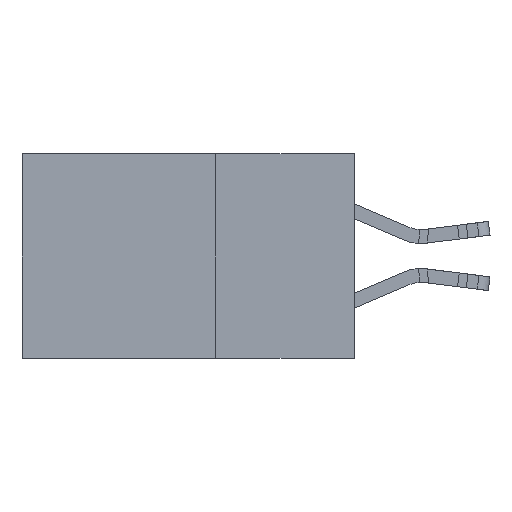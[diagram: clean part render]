
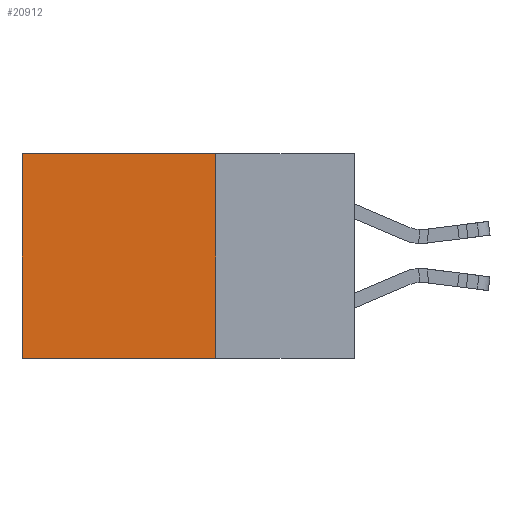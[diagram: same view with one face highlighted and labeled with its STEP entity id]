
A CAD part, left-side view. The second image highlights one B-rep face of the part: STEP entity #20912.
In plain terms, the highlighted planar face has unit normal (-1, 0, 0).
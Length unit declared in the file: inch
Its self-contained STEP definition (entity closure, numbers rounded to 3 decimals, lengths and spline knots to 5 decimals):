
#80 = VERTEX_POINT ( 'NONE', #6116 ) ;
#384 = LINE ( 'NONE', #6016, #4370 ) ;
#1955 = PLANE ( 'NONE',  #20661 ) ;
#1996 = VERTEX_POINT ( 'NONE', #16649 ) ;
#4211 = CARTESIAN_POINT ( 'NONE',  ( 0.2615, 0.25, 0. ) ) ;
#4322 = LINE ( 'NONE', #22541, #17549 ) ;
#4370 = VECTOR ( 'NONE', #15210, 39.37008 ) ;
#4405 = LINE ( 'NONE', #13364, #9918 ) ;
#5443 = FACE_OUTER_BOUND ( 'NONE', #13372, .T. ) ;
#6016 = CARTESIAN_POINT ( 'NONE',  ( 0.2615, 0.25, -0.37 ) ) ;
#6116 = CARTESIAN_POINT ( 'NONE',  ( 0.2615, 0.25, -0.37 ) ) ;
#7510 = CARTESIAN_POINT ( 'NONE',  ( 0.2615, 0.25, -0.37 ) ) ;
#7964 = DIRECTION ( 'NONE',  ( 0., 1., 0. ) ) ;
#8006 = VERTEX_POINT ( 'NONE', #10731 ) ;
#9540 = ORIENTED_EDGE ( 'NONE', *, *, #21520, .T. ) ;
#9557 = CARTESIAN_POINT ( 'NONE',  ( 0.2615, 0.25, 0. ) ) ;
#9918 = VECTOR ( 'NONE', #19125, 39.37008 ) ;
#10367 = ORIENTED_EDGE ( 'NONE', *, *, #22937, .T. ) ;
#10731 = CARTESIAN_POINT ( 'NONE',  ( 0.2615, 0.6, -0.37 ) ) ;
#13364 = CARTESIAN_POINT ( 'NONE',  ( 0.2615, 0.25, -0.37 ) ) ;
#13372 = EDGE_LOOP ( 'NONE', ( #9540, #13458, #20844, #10367 ) ) ;
#13458 = ORIENTED_EDGE ( 'NONE', *, *, #15633, .F. ) ;
#14982 = DIRECTION ( 'NONE',  ( 1., 0., 0. ) ) ;
#15204 = LINE ( 'NONE', #4211, #15698 ) ;
#15210 = DIRECTION ( 'NONE',  ( 0., 0., -1. ) ) ;
#15633 = EDGE_CURVE ( 'NONE', #80, #8006, #4405, .T. ) ;
#15698 = VECTOR ( 'NONE', #7964, 39.37008 ) ;
#16649 = CARTESIAN_POINT ( 'NONE',  ( 0.2615, 0.6, 0. ) ) ;
#17549 = VECTOR ( 'NONE', #22892, 39.37008 ) ;
#17566 = EDGE_CURVE ( 'NONE', #18889, #80, #384, .T. ) ;
#18889 = VERTEX_POINT ( 'NONE', #9557 ) ;
#19125 = DIRECTION ( 'NONE',  ( 0., 1., 0. ) ) ;
#20412 = DIRECTION ( 'NONE',  ( 0., 0., -1. ) ) ;
#20661 = AXIS2_PLACEMENT_3D ( 'NONE', #7510, #14982, #20412 ) ;
#20844 = ORIENTED_EDGE ( 'NONE', *, *, #17566, .F. ) ;
#20912 = ADVANCED_FACE ( 'NONE', ( #5443 ), #1955, .F. ) ;
#21520 = EDGE_CURVE ( 'NONE', #1996, #8006, #4322, .T. ) ;
#22541 = CARTESIAN_POINT ( 'NONE',  ( 0.2615, 0.6, -0.37 ) ) ;
#22892 = DIRECTION ( 'NONE',  ( 0., 0., -1. ) ) ;
#22937 = EDGE_CURVE ( 'NONE', #18889, #1996, #15204, .T. ) ;
